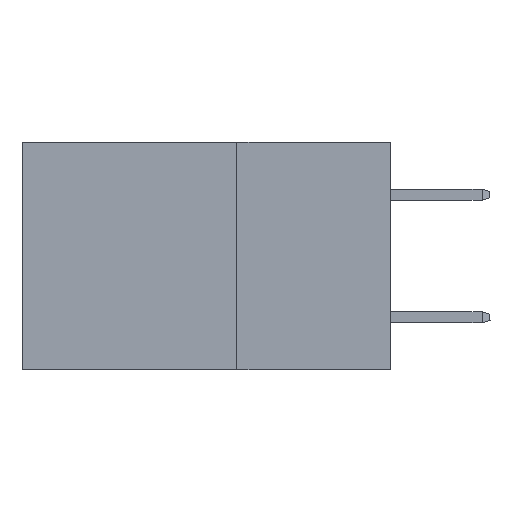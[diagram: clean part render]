
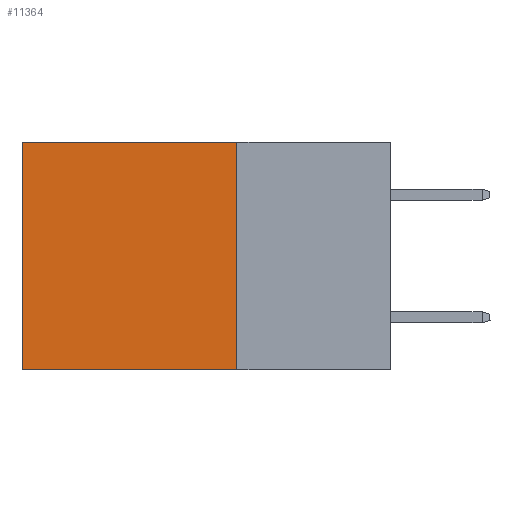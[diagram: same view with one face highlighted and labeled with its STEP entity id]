
A CAD part, left-side view. The second image highlights one B-rep face of the part: STEP entity #11364.
In plain terms, the highlighted planar face has unit normal (-1, 0, 0).
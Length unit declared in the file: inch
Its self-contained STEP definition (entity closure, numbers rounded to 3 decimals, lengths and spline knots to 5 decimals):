
#1272 = CARTESIAN_POINT ( 'NONE',  ( 0.2875, 0.25, -0.37 ) ) ;
#2561 = PLANE ( 'NONE',  #27730 ) ;
#6524 = ORIENTED_EDGE ( 'NONE', *, *, #20571, .F. ) ;
#6619 = DIRECTION ( 'NONE',  ( 0., 1., 0. ) ) ;
#7118 = DIRECTION ( 'NONE',  ( 0., 0., -1. ) ) ;
#7423 = DIRECTION ( 'NONE',  ( 1., 0., 0. ) ) ;
#9115 = CARTESIAN_POINT ( 'NONE',  ( 0.2875, 0.6, -0.37 ) ) ;
#9130 = CARTESIAN_POINT ( 'NONE',  ( 0.2875, 0.25, 0. ) ) ;
#9890 = VERTEX_POINT ( 'NONE', #18524 ) ;
#10868 = EDGE_CURVE ( 'NONE', #28198, #9890, #27509, .T. ) ;
#11364 = ADVANCED_FACE ( 'NONE', ( #20545 ), #2561, .F. ) ;
#11379 = DIRECTION ( 'NONE',  ( 0., 0., -1. ) ) ;
#11719 = VERTEX_POINT ( 'NONE', #9115 ) ;
#12282 = VERTEX_POINT ( 'NONE', #33601 ) ;
#13684 = CARTESIAN_POINT ( 'NONE',  ( 0.2875, 0.25, 0. ) ) ;
#14117 = VECTOR ( 'NONE', #32005, 39.37008 ) ;
#14978 = VECTOR ( 'NONE', #11379, 39.37008 ) ;
#15186 = CARTESIAN_POINT ( 'NONE',  ( 0.2875, 0.25, 0. ) ) ;
#15691 = DIRECTION ( 'NONE',  ( 0., 0., -1. ) ) ;
#16062 = EDGE_CURVE ( 'NONE', #28198, #12282, #21625, .T. ) ;
#18524 = CARTESIAN_POINT ( 'NONE',  ( 0.2875, 0.25, -0.37 ) ) ;
#19071 = ORIENTED_EDGE ( 'NONE', *, *, #16062, .T. ) ;
#20545 = FACE_OUTER_BOUND ( 'NONE', #22309, .T. ) ;
#20571 = EDGE_CURVE ( 'NONE', #9890, #11719, #21983, .T. ) ;
#21625 = LINE ( 'NONE', #13684, #14117 ) ;
#21896 = CARTESIAN_POINT ( 'NONE',  ( 0.2875, 0.6, 0. ) ) ;
#21983 = LINE ( 'NONE', #1272, #23085 ) ;
#22309 = EDGE_LOOP ( 'NONE', ( #29098, #6524, #23757, #19071 ) ) ;
#22826 = CARTESIAN_POINT ( 'NONE',  ( 0.2875, 0.25, 0. ) ) ;
#23085 = VECTOR ( 'NONE', #6619, 39.37008 ) ;
#23757 = ORIENTED_EDGE ( 'NONE', *, *, #10868, .F. ) ;
#24352 = VECTOR ( 'NONE', #7118, 39.37008 ) ;
#27269 = LINE ( 'NONE', #21896, #14978 ) ;
#27509 = LINE ( 'NONE', #22826, #24352 ) ;
#27730 = AXIS2_PLACEMENT_3D ( 'NONE', #15186, #7423, #15691 ) ;
#28198 = VERTEX_POINT ( 'NONE', #9130 ) ;
#29098 = ORIENTED_EDGE ( 'NONE', *, *, #32640, .T. ) ;
#32005 = DIRECTION ( 'NONE',  ( 0., 1., 0. ) ) ;
#32640 = EDGE_CURVE ( 'NONE', #12282, #11719, #27269, .T. ) ;
#33601 = CARTESIAN_POINT ( 'NONE',  ( 0.2875, 0.6, 0. ) ) ;
